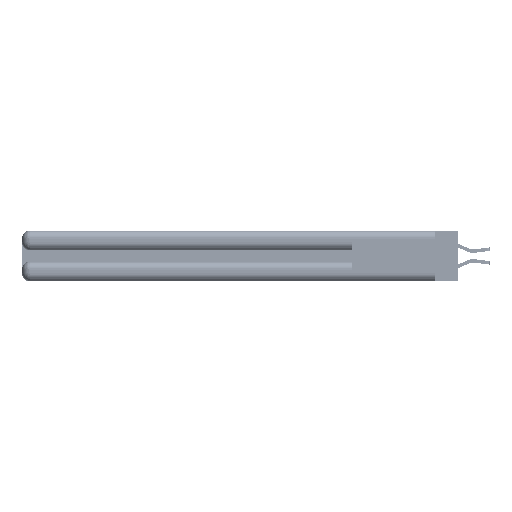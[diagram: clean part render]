
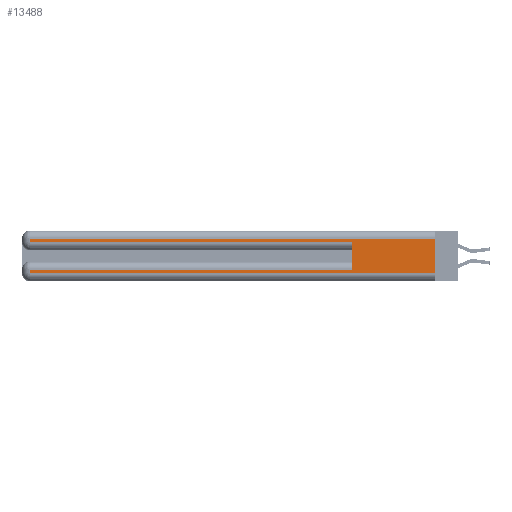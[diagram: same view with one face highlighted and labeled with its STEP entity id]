
A CAD part, left-side view. The second image highlights one B-rep face of the part: STEP entity #13488.
In plain terms, the highlighted planar face has unit normal (-1, 0, 0).
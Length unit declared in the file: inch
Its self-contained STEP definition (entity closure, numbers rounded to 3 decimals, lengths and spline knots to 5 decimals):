
#331 = ORIENTED_EDGE ( 'NONE', *, *, #4156, .T. ) ;
#2140 = DIRECTION ( 'NONE',  ( 1., 0., 0. ) ) ;
#3556 = ORIENTED_EDGE ( 'NONE', *, *, #8047, .F. ) ;
#4116 = DIRECTION ( 'NONE',  ( 0., 1., 0. ) ) ;
#4156 = EDGE_CURVE ( 'NONE', #8421, #20161, #10604, .T. ) ;
#5152 = VECTOR ( 'NONE', #46531, 39.37008 ) ;
#5178 = DIRECTION ( 'NONE',  ( 0., 0., -1. ) ) ;
#6581 = VECTOR ( 'NONE', #4116, 39.37008 ) ;
#7047 = VECTOR ( 'NONE', #42127, 39.37008 ) ;
#7755 = VECTOR ( 'NONE', #5178, 39.37008 ) ;
#7873 = CARTESIAN_POINT ( 'NONE',  ( 0., 0., 0.085 ) ) ;
#8047 = EDGE_CURVE ( 'NONE', #8421, #28577, #28423, .T. ) ;
#8421 = VERTEX_POINT ( 'NONE', #16745 ) ;
#10604 = LINE ( 'NONE', #10824, #25173 ) ;
#10824 = CARTESIAN_POINT ( 'NONE',  ( 0., 0., 0.31 ) ) ;
#11136 = ORIENTED_EDGE ( 'NONE', *, *, #34554, .T. ) ;
#12218 = CARTESIAN_POINT ( 'NONE',  ( 0., 0., 0.06 ) ) ;
#12675 = DIRECTION ( 'NONE',  ( 0., 0., 1. ) ) ;
#13488 = ADVANCED_FACE ( 'NONE', ( #47307 ), #45096, .F. ) ;
#16174 = CARTESIAN_POINT ( 'NONE',  ( 0., 2.94, 0.06 ) ) ;
#16363 = CARTESIAN_POINT ( 'NONE',  ( 0., 0., 0.37 ) ) ;
#16514 = VERTEX_POINT ( 'NONE', #38741 ) ;
#16745 = CARTESIAN_POINT ( 'NONE',  ( 0., 0., 0.31 ) ) ;
#18177 = DIRECTION ( 'NONE',  ( 0., -1., 0. ) ) ;
#18216 = EDGE_CURVE ( 'NONE', #46040, #49696, #48562, .T. ) ;
#20161 = VERTEX_POINT ( 'NONE', #46759 ) ;
#20171 = EDGE_CURVE ( 'NONE', #47391, #46040, #37543, .T. ) ;
#21135 = ORIENTED_EDGE ( 'NONE', *, *, #45958, .T. ) ;
#21783 = EDGE_CURVE ( 'NONE', #47391, #30976, #47129, .T. ) ;
#22717 = DIRECTION ( 'NONE',  ( 0., 1., 0. ) ) ;
#24719 = CARTESIAN_POINT ( 'NONE',  ( 0., 0.6, 0.145 ) ) ;
#24731 = ORIENTED_EDGE ( 'NONE', *, *, #33674, .T. ) ;
#25173 = VECTOR ( 'NONE', #22717, 39.37008 ) ;
#27032 = LINE ( 'NONE', #12218, #5152 ) ;
#27347 = CARTESIAN_POINT ( 'NONE',  ( 0., 0., 0.06 ) ) ;
#28423 = LINE ( 'NONE', #16363, #7755 ) ;
#28577 = VERTEX_POINT ( 'NONE', #27347 ) ;
#28674 = AXIS2_PLACEMENT_3D ( 'NONE', #33055, #2140, #33565 ) ;
#29708 = LINE ( 'NONE', #31515, #34564 ) ;
#30976 = VERTEX_POINT ( 'NONE', #45221 ) ;
#31515 = CARTESIAN_POINT ( 'NONE',  ( 0., 2.94, 0.37 ) ) ;
#32307 = CARTESIAN_POINT ( 'NONE',  ( 0., 0.6, 0.085 ) ) ;
#33055 = CARTESIAN_POINT ( 'NONE',  ( 0., 0., 0.37 ) ) ;
#33472 = ORIENTED_EDGE ( 'NONE', *, *, #20171, .T. ) ;
#33565 = DIRECTION ( 'NONE',  ( 0., 0., -1. ) ) ;
#33674 = EDGE_CURVE ( 'NONE', #16514, #30976, #38902, .T. ) ;
#33755 = VECTOR ( 'NONE', #12675, 39.37008 ) ;
#34554 = EDGE_CURVE ( 'NONE', #20161, #16514, #29708, .T. ) ;
#34564 = VECTOR ( 'NONE', #40291, 39.37008 ) ;
#37543 = LINE ( 'NONE', #7873, #6581 ) ;
#38741 = CARTESIAN_POINT ( 'NONE',  ( 0., 2.94, 0.285 ) ) ;
#38902 = LINE ( 'NONE', #45685, #40722 ) ;
#40291 = DIRECTION ( 'NONE',  ( 0., 0., -1. ) ) ;
#40722 = VECTOR ( 'NONE', #18177, 39.37008 ) ;
#41414 = ORIENTED_EDGE ( 'NONE', *, *, #21783, .F. ) ;
#42127 = DIRECTION ( 'NONE',  ( 0., 0., -1. ) ) ;
#43112 = CARTESIAN_POINT ( 'NONE',  ( 0., 2.94, 0.085 ) ) ;
#43139 = ORIENTED_EDGE ( 'NONE', *, *, #18216, .T. ) ;
#45096 = PLANE ( 'NONE',  #28674 ) ;
#45221 = CARTESIAN_POINT ( 'NONE',  ( 0., 0.6, 0.285 ) ) ;
#45678 = EDGE_LOOP ( 'NONE', ( #3556, #331, #11136, #24731, #41414, #33472, #43139, #21135 ) ) ;
#45685 = CARTESIAN_POINT ( 'NONE',  ( 0., 0., 0.285 ) ) ;
#45730 = CARTESIAN_POINT ( 'NONE',  ( 0., 2.94, 0.37 ) ) ;
#45958 = EDGE_CURVE ( 'NONE', #49696, #28577, #27032, .T. ) ;
#46040 = VERTEX_POINT ( 'NONE', #43112 ) ;
#46531 = DIRECTION ( 'NONE',  ( 0., -1., 0. ) ) ;
#46759 = CARTESIAN_POINT ( 'NONE',  ( 0., 2.94, 0.31 ) ) ;
#47129 = LINE ( 'NONE', #24719, #33755 ) ;
#47307 = FACE_OUTER_BOUND ( 'NONE', #45678, .T. ) ;
#47391 = VERTEX_POINT ( 'NONE', #32307 ) ;
#48562 = LINE ( 'NONE', #45730, #7047 ) ;
#49696 = VERTEX_POINT ( 'NONE', #16174 ) ;
